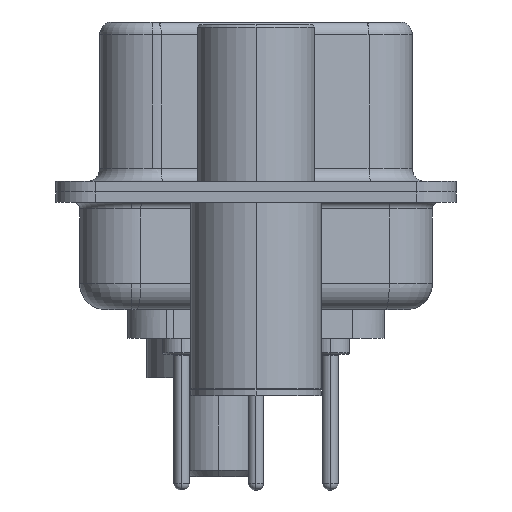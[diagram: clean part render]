
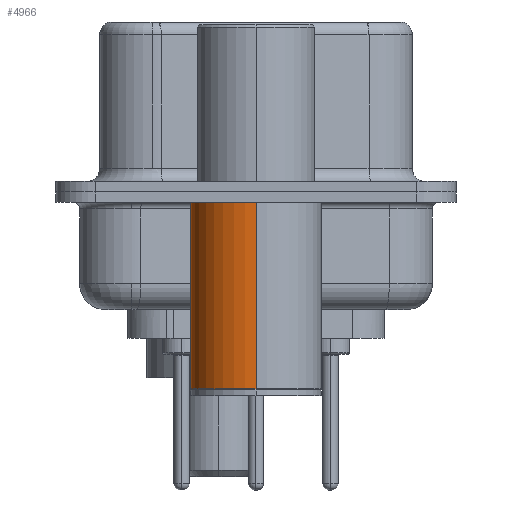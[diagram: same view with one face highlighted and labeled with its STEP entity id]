
A CAD part, left-side view. The second image highlights one B-rep face of the part: STEP entity #4966.
In plain terms, the highlighted cylindrical face has radius 2.5 mm (diameter 5 mm), a partial arc.
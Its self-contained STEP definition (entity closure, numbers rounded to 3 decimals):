
#1557 = ORIENTED_EDGE ( 'NONE', *, *, #4920, .T. ) ;
#2672 = CYLINDRICAL_SURFACE ( 'NONE', #16703, 2.5 ) ;
#3506 = CARTESIAN_POINT ( 'NONE',  ( 2.5, 0., -0.4 ) ) ;
#3822 = AXIS2_PLACEMENT_3D ( 'NONE', #6459, #26953, #30357 ) ;
#4207 = VECTOR ( 'NONE', #21184, 1000. ) ;
#4336 = CARTESIAN_POINT ( 'NONE',  ( 2.5, 0., 0.581 ) ) ;
#4920 = EDGE_CURVE ( 'NONE', #22900, #8755, #9901, .T. ) ;
#4966 = ADVANCED_FACE ( 'NONE', ( #22675 ), #2672, .T. ) ;
#5437 = CARTESIAN_POINT ( 'NONE',  ( -2.5, 0., 0.581 ) ) ;
#5752 = AXIS2_PLACEMENT_3D ( 'NONE', #21549, #7102, #23969 ) ;
#6459 = CARTESIAN_POINT ( 'NONE',  ( 0., 0., -7.525 ) ) ;
#7102 = DIRECTION ( 'NONE',  ( 0., 0., 1. ) ) ;
#7561 = ORIENTED_EDGE ( 'NONE', *, *, #20455, .F. ) ;
#7598 = VECTOR ( 'NONE', #19878, 1000. ) ;
#8755 = VERTEX_POINT ( 'NONE', #10662 ) ;
#9901 = CIRCLE ( 'NONE', #3822, 2.5 ) ;
#9967 = DIRECTION ( 'NONE',  ( 0., 0., 1. ) ) ;
#10662 = CARTESIAN_POINT ( 'NONE',  ( -2.5, 0., -7.525 ) ) ;
#12321 = VERTEX_POINT ( 'NONE', #13703 ) ;
#13415 = ORIENTED_EDGE ( 'NONE', *, *, #30700, .T. ) ;
#13703 = CARTESIAN_POINT ( 'NONE',  ( -2.5, 0., -0.4 ) ) ;
#16555 = VERTEX_POINT ( 'NONE', #3506 ) ;
#16703 = AXIS2_PLACEMENT_3D ( 'NONE', #23871, #9967, #23903 ) ;
#16923 = CIRCLE ( 'NONE', #5752, 2.5 ) ;
#19878 = DIRECTION ( 'NONE',  ( 0., 0., 1. ) ) ;
#20402 = LINE ( 'NONE', #5437, #7598 ) ;
#20455 = EDGE_CURVE ( 'NONE', #16555, #12321, #16923, .T. ) ;
#20996 = EDGE_LOOP ( 'NONE', ( #1557, #13415, #7561, #30613 ) ) ;
#21184 = DIRECTION ( 'NONE',  ( 0., 0., 1. ) ) ;
#21549 = CARTESIAN_POINT ( 'NONE',  ( 0., 0., -0.4 ) ) ;
#22675 = FACE_OUTER_BOUND ( 'NONE', #20996, .T. ) ;
#22900 = VERTEX_POINT ( 'NONE', #29715 ) ;
#23681 = EDGE_CURVE ( 'NONE', #22900, #16555, #24192, .T. ) ;
#23871 = CARTESIAN_POINT ( 'NONE',  ( 0., 0., 0.581 ) ) ;
#23903 = DIRECTION ( 'NONE',  ( 1., 0., 0. ) ) ;
#23969 = DIRECTION ( 'NONE',  ( 1., 0., 0. ) ) ;
#24192 = LINE ( 'NONE', #4336, #4207 ) ;
#26953 = DIRECTION ( 'NONE',  ( 0., 0., 1. ) ) ;
#29715 = CARTESIAN_POINT ( 'NONE',  ( 2.5, 0., -7.525 ) ) ;
#30357 = DIRECTION ( 'NONE',  ( 1., 0., 0. ) ) ;
#30613 = ORIENTED_EDGE ( 'NONE', *, *, #23681, .F. ) ;
#30700 = EDGE_CURVE ( 'NONE', #8755, #12321, #20402, .T. ) ;
